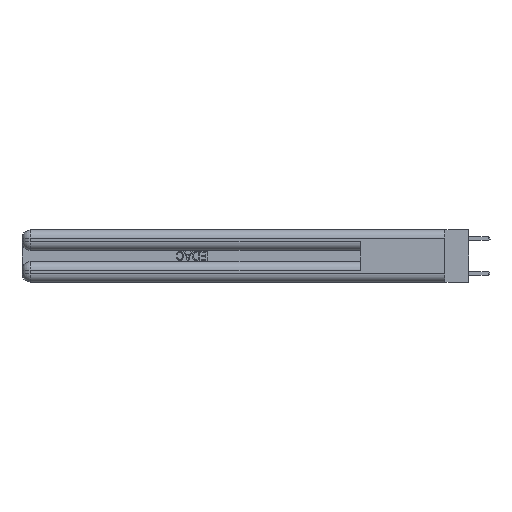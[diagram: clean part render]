
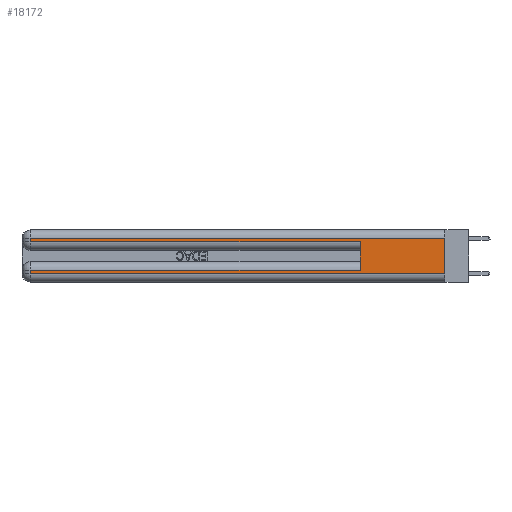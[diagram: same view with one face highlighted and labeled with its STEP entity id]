
A CAD part, left-side view. The second image highlights one B-rep face of the part: STEP entity #18172.
In plain terms, the highlighted planar face has unit normal (-1, 0, 0).
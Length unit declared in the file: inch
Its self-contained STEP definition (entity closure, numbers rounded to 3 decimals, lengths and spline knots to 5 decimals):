
#673 = ORIENTED_EDGE ( 'NONE', *, *, #9799, .T. ) ;
#716 = LINE ( 'NONE', #5538, #11797 ) ;
#827 = DIRECTION ( 'NONE',  ( 0., -1., 0. ) ) ;
#1192 = VERTEX_POINT ( 'NONE', #9352 ) ;
#1722 = LINE ( 'NONE', #20560, #23589 ) ;
#1873 = DIRECTION ( 'NONE',  ( 0., 1., 0. ) ) ;
#2753 = VERTEX_POINT ( 'NONE', #4636 ) ;
#3316 = VERTEX_POINT ( 'NONE', #15108 ) ;
#3470 = CARTESIAN_POINT ( 'NONE',  ( 0., 2.94, 0.06 ) ) ;
#4045 = PLANE ( 'NONE',  #17591 ) ;
#4083 = VERTEX_POINT ( 'NONE', #20541 ) ;
#4169 = CARTESIAN_POINT ( 'NONE',  ( 0., 2.94, 0.285 ) ) ;
#4636 = CARTESIAN_POINT ( 'NONE',  ( 0., 0.6, 0.285 ) ) ;
#5192 = VERTEX_POINT ( 'NONE', #4169 ) ;
#5538 = CARTESIAN_POINT ( 'NONE',  ( 0., 0., 0.37 ) ) ;
#5556 = VERTEX_POINT ( 'NONE', #3470 ) ;
#5790 = EDGE_LOOP ( 'NONE', ( #10359, #8042, #25785, #18972, #17392, #21671, #8797, #673 ) ) ;
#6013 = LINE ( 'NONE', #10126, #10467 ) ;
#6273 = EDGE_CURVE ( 'NONE', #1192, #5556, #22341, .T. ) ;
#6299 = CARTESIAN_POINT ( 'NONE',  ( 0., 0., 0.085 ) ) ;
#6864 = DIRECTION ( 'NONE',  ( 0., 0., -1. ) ) ;
#7450 = EDGE_CURVE ( 'NONE', #9042, #3316, #716, .T. ) ;
#7610 = DIRECTION ( 'NONE',  ( 0., -1., 0. ) ) ;
#7780 = DIRECTION ( 'NONE',  ( 0., 0., -1. ) ) ;
#7804 = VERTEX_POINT ( 'NONE', #15836 ) ;
#8042 = ORIENTED_EDGE ( 'NONE', *, *, #9497, .T. ) ;
#8550 = CARTESIAN_POINT ( 'NONE',  ( 0., 0., 0.37 ) ) ;
#8730 = LINE ( 'NONE', #13023, #19538 ) ;
#8797 = ORIENTED_EDGE ( 'NONE', *, *, #6273, .T. ) ;
#9042 = VERTEX_POINT ( 'NONE', #15697 ) ;
#9352 = CARTESIAN_POINT ( 'NONE',  ( 0., 2.94, 0.085 ) ) ;
#9497 = EDGE_CURVE ( 'NONE', #9042, #7804, #8730, .T. ) ;
#9799 = EDGE_CURVE ( 'NONE', #5556, #3316, #1722, .T. ) ;
#10126 = CARTESIAN_POINT ( 'NONE',  ( 0., 0.6, 0.145 ) ) ;
#10359 = ORIENTED_EDGE ( 'NONE', *, *, #7450, .F. ) ;
#10467 = VECTOR ( 'NONE', #16647, 39.37008 ) ;
#10699 = DIRECTION ( 'NONE',  ( 1., 0., 0. ) ) ;
#10832 = DIRECTION ( 'NONE',  ( 0., 1., 0. ) ) ;
#10927 = LINE ( 'NONE', #22638, #11622 ) ;
#11527 = EDGE_CURVE ( 'NONE', #4083, #1192, #27150, .T. ) ;
#11622 = VECTOR ( 'NONE', #827, 39.37008 ) ;
#11797 = VECTOR ( 'NONE', #7780, 39.37008 ) ;
#13023 = CARTESIAN_POINT ( 'NONE',  ( 0., 0., 0.31 ) ) ;
#13765 = EDGE_CURVE ( 'NONE', #7804, #5192, #21043, .T. ) ;
#15108 = CARTESIAN_POINT ( 'NONE',  ( 0., 0., 0.06 ) ) ;
#15293 = EDGE_CURVE ( 'NONE', #4083, #2753, #6013, .T. ) ;
#15697 = CARTESIAN_POINT ( 'NONE',  ( 0., 0., 0.31 ) ) ;
#15748 = VECTOR ( 'NONE', #1873, 39.37008 ) ;
#15836 = CARTESIAN_POINT ( 'NONE',  ( 0., 2.94, 0.31 ) ) ;
#16607 = VECTOR ( 'NONE', #19001, 39.37008 ) ;
#16647 = DIRECTION ( 'NONE',  ( 0., 0., 1. ) ) ;
#16843 = CARTESIAN_POINT ( 'NONE',  ( 0., 2.94, 0.37 ) ) ;
#17392 = ORIENTED_EDGE ( 'NONE', *, *, #15293, .F. ) ;
#17591 = AXIS2_PLACEMENT_3D ( 'NONE', #8550, #10699, #25765 ) ;
#17679 = CARTESIAN_POINT ( 'NONE',  ( 0., 2.94, 0.37 ) ) ;
#18172 = ADVANCED_FACE ( 'NONE', ( #23637 ), #4045, .F. ) ;
#18972 = ORIENTED_EDGE ( 'NONE', *, *, #21982, .T. ) ;
#19001 = DIRECTION ( 'NONE',  ( 0., 0., -1. ) ) ;
#19538 = VECTOR ( 'NONE', #10832, 39.37008 ) ;
#20350 = VECTOR ( 'NONE', #6864, 39.37008 ) ;
#20541 = CARTESIAN_POINT ( 'NONE',  ( 0., 0.6, 0.085 ) ) ;
#20560 = CARTESIAN_POINT ( 'NONE',  ( 0., 0., 0.06 ) ) ;
#21043 = LINE ( 'NONE', #17679, #20350 ) ;
#21671 = ORIENTED_EDGE ( 'NONE', *, *, #11527, .T. ) ;
#21982 = EDGE_CURVE ( 'NONE', #5192, #2753, #10927, .T. ) ;
#22341 = LINE ( 'NONE', #16843, #16607 ) ;
#22638 = CARTESIAN_POINT ( 'NONE',  ( 0., 0., 0.285 ) ) ;
#23589 = VECTOR ( 'NONE', #7610, 39.37008 ) ;
#23637 = FACE_OUTER_BOUND ( 'NONE', #5790, .T. ) ;
#25765 = DIRECTION ( 'NONE',  ( 0., 0., -1. ) ) ;
#25785 = ORIENTED_EDGE ( 'NONE', *, *, #13765, .T. ) ;
#27150 = LINE ( 'NONE', #6299, #15748 ) ;
